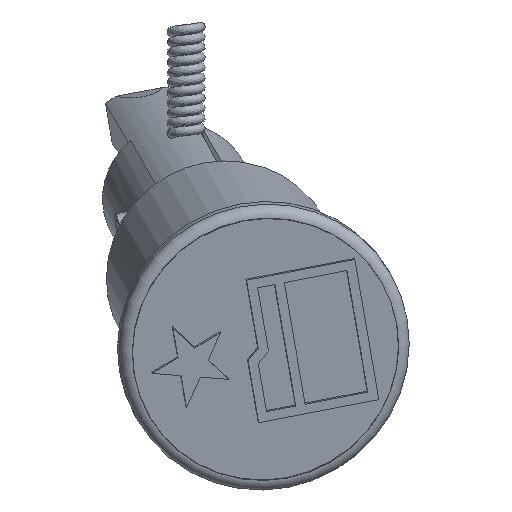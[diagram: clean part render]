
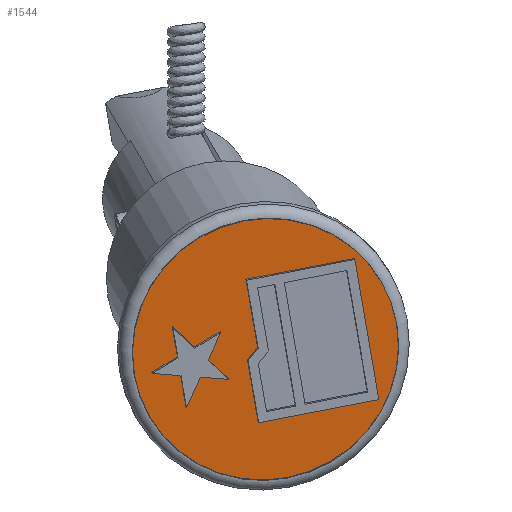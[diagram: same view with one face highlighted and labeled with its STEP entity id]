
A CAD part, top view. The second image highlights one B-rep face of the part: STEP entity #1544.
In plain terms, the highlighted face is planar.
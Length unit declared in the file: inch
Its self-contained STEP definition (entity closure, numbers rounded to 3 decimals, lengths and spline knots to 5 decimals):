
#92=FACE_BOUND('',#277,.T.);
#93=FACE_BOUND('',#278,.T.);
#116=CIRCLE('',#1756,0.277);
#183=FACE_OUTER_BOUND('',#276,.T.);
#276=EDGE_LOOP('',(#1066));
#277=EDGE_LOOP('',(#1067,#1068,#1069,#1070,#1071,#1072));
#278=EDGE_LOOP('',(#1073,#1074,#1075,#1076,#1077,#1078,#1079,#1080,#1081,
#1082));
#402=LINE('',#2405,#551);
#403=LINE('',#2407,#552);
#404=LINE('',#2409,#553);
#405=LINE('',#2411,#554);
#406=LINE('',#2413,#555);
#407=LINE('',#2414,#556);
#408=LINE('',#2417,#557);
#409=LINE('',#2419,#558);
#410=LINE('',#2421,#559);
#411=LINE('',#2423,#560);
#412=LINE('',#2425,#561);
#413=LINE('',#2427,#562);
#414=LINE('',#2429,#563);
#415=LINE('',#2431,#564);
#416=LINE('',#2433,#565);
#417=LINE('',#2434,#566);
#551=VECTOR('',#1939,0.3937);
#552=VECTOR('',#1940,0.3937);
#553=VECTOR('',#1941,0.3937);
#554=VECTOR('',#1942,0.3937);
#555=VECTOR('',#1943,0.3937);
#556=VECTOR('',#1944,0.3937);
#557=VECTOR('',#1945,0.3937);
#558=VECTOR('',#1946,0.3937);
#559=VECTOR('',#1947,0.3937);
#560=VECTOR('',#1948,0.3937);
#561=VECTOR('',#1949,0.3937);
#562=VECTOR('',#1950,0.3937);
#563=VECTOR('',#1951,0.3937);
#564=VECTOR('',#1952,0.3937);
#565=VECTOR('',#1953,0.3937);
#566=VECTOR('',#1954,0.3937);
#698=VERTEX_POINT('',#2398);
#700=VERTEX_POINT('',#2403);
#701=VERTEX_POINT('',#2404);
#702=VERTEX_POINT('',#2406);
#703=VERTEX_POINT('',#2408);
#704=VERTEX_POINT('',#2410);
#705=VERTEX_POINT('',#2412);
#706=VERTEX_POINT('',#2415);
#707=VERTEX_POINT('',#2416);
#708=VERTEX_POINT('',#2418);
#709=VERTEX_POINT('',#2420);
#710=VERTEX_POINT('',#2422);
#711=VERTEX_POINT('',#2424);
#712=VERTEX_POINT('',#2426);
#713=VERTEX_POINT('',#2428);
#714=VERTEX_POINT('',#2430);
#715=VERTEX_POINT('',#2432);
#849=EDGE_CURVE('',#698,#698,#116,.T.);
#851=EDGE_CURVE('',#700,#701,#402,.T.);
#852=EDGE_CURVE('',#702,#700,#403,.T.);
#853=EDGE_CURVE('',#703,#702,#404,.T.);
#854=EDGE_CURVE('',#704,#703,#405,.T.);
#855=EDGE_CURVE('',#705,#704,#406,.T.);
#856=EDGE_CURVE('',#701,#705,#407,.T.);
#857=EDGE_CURVE('',#706,#707,#408,.T.);
#858=EDGE_CURVE('',#708,#706,#409,.T.);
#859=EDGE_CURVE('',#709,#708,#410,.T.);
#860=EDGE_CURVE('',#710,#709,#411,.T.);
#861=EDGE_CURVE('',#711,#710,#412,.T.);
#862=EDGE_CURVE('',#712,#711,#413,.T.);
#863=EDGE_CURVE('',#713,#712,#414,.T.);
#864=EDGE_CURVE('',#714,#713,#415,.T.);
#865=EDGE_CURVE('',#715,#714,#416,.T.);
#866=EDGE_CURVE('',#707,#715,#417,.T.);
#1066=ORIENTED_EDGE('',*,*,#849,.F.);
#1067=ORIENTED_EDGE('',*,*,#851,.F.);
#1068=ORIENTED_EDGE('',*,*,#852,.F.);
#1069=ORIENTED_EDGE('',*,*,#853,.F.);
#1070=ORIENTED_EDGE('',*,*,#854,.F.);
#1071=ORIENTED_EDGE('',*,*,#855,.F.);
#1072=ORIENTED_EDGE('',*,*,#856,.F.);
#1073=ORIENTED_EDGE('',*,*,#857,.F.);
#1074=ORIENTED_EDGE('',*,*,#858,.F.);
#1075=ORIENTED_EDGE('',*,*,#859,.F.);
#1076=ORIENTED_EDGE('',*,*,#860,.F.);
#1077=ORIENTED_EDGE('',*,*,#861,.F.);
#1078=ORIENTED_EDGE('',*,*,#862,.F.);
#1079=ORIENTED_EDGE('',*,*,#863,.F.);
#1080=ORIENTED_EDGE('',*,*,#864,.F.);
#1081=ORIENTED_EDGE('',*,*,#865,.F.);
#1082=ORIENTED_EDGE('',*,*,#866,.F.);
#1474=PLANE('',#1758);
#1544=ADVANCED_FACE('',(#183,#92,#93),#1474,.T.);
#1756=AXIS2_PLACEMENT_3D('',#2399,#1933,#1934);
#1758=AXIS2_PLACEMENT_3D('',#2402,#1937,#1938);
#1933=DIRECTION('center_axis',(0.,0.,-1.));
#1934=DIRECTION('ref_axis',(-1.,0.,0.));
#1937=DIRECTION('center_axis',(0.,0.,1.));
#1938=DIRECTION('ref_axis',(1.,0.,0.));
#1939=DIRECTION('',(-1.,0.,0.));
#1940=DIRECTION('',(0.,1.,0.));
#1941=DIRECTION('',(1.,0.,0.));
#1942=DIRECTION('',(0.,-1.,0.));
#1943=DIRECTION('',(-0.765,-0.645,0.));
#1944=DIRECTION('',(0.,-1.,0.));
#1945=DIRECTION('',(0.,-1.,0.));
#1946=DIRECTION('',(-0.593,0.805,0.));
#1947=DIRECTION('',(-0.937,-0.349,0.));
#1948=DIRECTION('',(0.559,0.829,0.));
#1949=DIRECTION('',(-0.593,0.805,0.));
#1950=DIRECTION('',(0.963,-0.269,0.));
#1951=DIRECTION('',(0.559,0.829,0.));
#1952=DIRECTION('',(0.,-1.,0.));
#1953=DIRECTION('',(0.963,-0.269,0.));
#1954=DIRECTION('',(-0.937,-0.349,0.));
#2398=CARTESIAN_POINT('',(0.277,0.,0.708));
#2399=CARTESIAN_POINT('Origin',(0.,0.,0.708));
#2402=CARTESIAN_POINT('Origin',(0.,0.,
0.708));
#2403=CARTESIAN_POINT('',(0.21334,0.15319,0.708));
#2404=CARTESIAN_POINT('',(-0.01512,0.15319,0.708));
#2405=CARTESIAN_POINT('',(-0.00756,0.15319,0.708));
#2406=CARTESIAN_POINT('',(0.21334,-0.14878,0.708));
#2407=CARTESIAN_POINT('',(0.21334,0.0766,0.708));
#2408=CARTESIAN_POINT('',(-0.04028,-0.14878,0.708));
#2409=CARTESIAN_POINT('',(0.10667,-0.14878,0.708));
#2410=CARTESIAN_POINT('',(-0.04028,-0.01489,0.708));
#2411=CARTESIAN_POINT('',(-0.04028,-0.07439,0.708));
#2412=CARTESIAN_POINT('',(-0.01512,0.00633,0.708));
#2413=CARTESIAN_POINT('',(-0.02484,-0.00187,0.708));
#2414=CARTESIAN_POINT('',(-0.01512,0.00316,0.708));
#2415=CARTESIAN_POINT('',(-0.18236,0.08433,0.708));
#2416=CARTESIAN_POINT('',(-0.18236,0.0187,0.708));
#2417=CARTESIAN_POINT('',(-0.18236,0.00935,0.708));
#2418=CARTESIAN_POINT('',(-0.14442,0.03282,0.708));
#2419=CARTESIAN_POINT('',(-0.13016,0.01345,0.708));
#2420=CARTESIAN_POINT('',(-0.08627,0.05447,0.708));
#2421=CARTESIAN_POINT('',(-0.08637,0.05444,0.708));
#2422=CARTESIAN_POINT('',(-0.12168,0.00194,0.708));
#2423=CARTESIAN_POINT('',(-0.08541,0.05574,0.708));
#2424=CARTESIAN_POINT('',(-0.08627,-0.04614,0.708));
#2425=CARTESIAN_POINT('',(-0.09982,-0.02774,0.708));
#2426=CARTESIAN_POINT('',(-0.14334,-0.03018,0.708));
#2427=CARTESIAN_POINT('',(-0.05225,-0.05566,0.708));
#2428=CARTESIAN_POINT('',(-0.18236,-0.08806,0.708));
#2429=CARTESIAN_POINT('',(-0.11395,0.01342,0.708));
#2430=CARTESIAN_POINT('',(-0.18236,-0.01926,0.708));
#2431=CARTESIAN_POINT('',(-0.18236,-0.04403,0.708));
#2432=CARTESIAN_POINT('',(-0.24056,-0.00297,0.708));
#2433=CARTESIAN_POINT('',(-0.1003,-0.04222,0.708));
#2434=CARTESIAN_POINT('',(-0.13444,0.03654,0.708));
